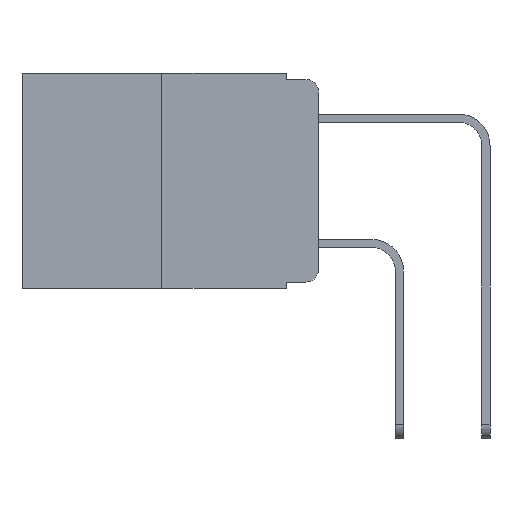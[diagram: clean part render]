
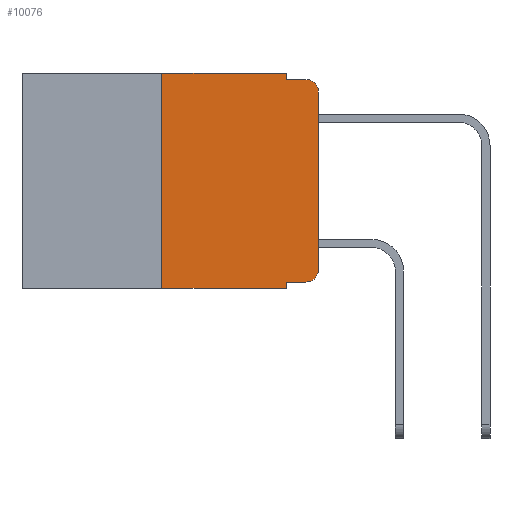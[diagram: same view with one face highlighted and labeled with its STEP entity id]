
A CAD part, left-side view. The second image highlights one B-rep face of the part: STEP entity #10076.
In plain terms, the highlighted planar face has unit normal (-1, 0, 0).
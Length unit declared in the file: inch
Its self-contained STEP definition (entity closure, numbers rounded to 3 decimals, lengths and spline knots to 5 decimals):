
#335 = DIRECTION ( 'NONE',  ( 0., -1., 0. ) ) ;
#600 = VERTEX_POINT ( 'NONE', #12245 ) ;
#879 = VERTEX_POINT ( 'NONE', #8091 ) ;
#1164 = VECTOR ( 'NONE', #9520, 39.37008 ) ;
#1260 = EDGE_CURVE ( 'NONE', #3278, #600, #9013, .T. ) ;
#1287 = CARTESIAN_POINT ( 'NONE',  ( 0., 0.051, 0. ) ) ;
#1298 = LINE ( 'NONE', #4380, #4053 ) ;
#1307 = VECTOR ( 'NONE', #12682, 39.37008 ) ;
#1690 = ORIENTED_EDGE ( 'NONE', *, *, #4685, .F. ) ;
#1772 = PLANE ( 'NONE',  #10299 ) ;
#1871 = CARTESIAN_POINT ( 'NONE',  ( 0., 0.02, -0.03 ) ) ;
#1982 = EDGE_CURVE ( 'NONE', #11834, #3278, #9294, .T. ) ;
#2088 = ORIENTED_EDGE ( 'NONE', *, *, #6685, .T. ) ;
#2178 = ORIENTED_EDGE ( 'NONE', *, *, #5344, .T. ) ;
#2198 = DIRECTION ( 'NONE',  ( -1., 0., 0. ) ) ;
#2210 = CARTESIAN_POINT ( 'NONE',  ( 0., 0.02, -0.313 ) ) ;
#2483 = CARTESIAN_POINT ( 'NONE',  ( 0., 0.25, 0. ) ) ;
#2591 = ORIENTED_EDGE ( 'NONE', *, *, #5039, .F. ) ;
#2690 = ORIENTED_EDGE ( 'NONE', *, *, #4041, .F. ) ;
#2692 = EDGE_CURVE ( 'NONE', #11834, #7189, #11748, .T. ) ;
#2758 = CARTESIAN_POINT ( 'NONE',  ( 0., 0.051, -0.333 ) ) ;
#2781 = ORIENTED_EDGE ( 'NONE', *, *, #1260, .T. ) ;
#2827 = EDGE_LOOP ( 'NONE', ( #2088, #2178, #1690, #2690, #2591, #6445, #5097, #8397, #3739, #2781 ) ) ;
#2858 = CARTESIAN_POINT ( 'NONE',  ( 0., 0.473, 0. ) ) ;
#2954 = DIRECTION ( 'NONE',  ( 0., 0., -1. ) ) ;
#3278 = VERTEX_POINT ( 'NONE', #11282 ) ;
#3390 = EDGE_CURVE ( 'NONE', #12925, #11996, #3933, .T. ) ;
#3414 = DIRECTION ( 'NONE',  ( 0., 0., -1. ) ) ;
#3492 = CARTESIAN_POINT ( 'NONE',  ( 0., 0.473, -0.343 ) ) ;
#3495 = VERTEX_POINT ( 'NONE', #11625 ) ;
#3739 = ORIENTED_EDGE ( 'NONE', *, *, #1982, .T. ) ;
#3858 = DIRECTION ( 'NONE',  ( 1., 0., 0. ) ) ;
#3933 = LINE ( 'NONE', #2483, #1164 ) ;
#3936 = CARTESIAN_POINT ( 'NONE',  ( 0., 0.051, 0. ) ) ;
#4041 = EDGE_CURVE ( 'NONE', #8054, #4931, #6684, .T. ) ;
#4053 = VECTOR ( 'NONE', #10375, 39.37008 ) ;
#4326 = CARTESIAN_POINT ( 'NONE',  ( 0., 0.051, -0.343 ) ) ;
#4380 = CARTESIAN_POINT ( 'NONE',  ( 0., 0.473, 0. ) ) ;
#4685 = EDGE_CURVE ( 'NONE', #4931, #879, #11849, .T. ) ;
#4931 = VERTEX_POINT ( 'NONE', #11191 ) ;
#5018 = CARTESIAN_POINT ( 'NONE',  ( 0., 0.25, 0. ) ) ;
#5039 = EDGE_CURVE ( 'NONE', #11996, #8054, #1298, .T. ) ;
#5097 = ORIENTED_EDGE ( 'NONE', *, *, #12477, .T. ) ;
#5344 = EDGE_CURVE ( 'NONE', #3495, #879, #10301, .T. ) ;
#5357 = CARTESIAN_POINT ( 'NONE',  ( 0., 0.25, -0.343 ) ) ;
#6403 = VECTOR ( 'NONE', #3414, 39.37008 ) ;
#6445 = ORIENTED_EDGE ( 'NONE', *, *, #3390, .F. ) ;
#6581 = VECTOR ( 'NONE', #10231, 39.37008 ) ;
#6684 = LINE ( 'NONE', #12639, #1307 ) ;
#6685 = EDGE_CURVE ( 'NONE', #600, #3495, #10144, .T. ) ;
#7189 = VERTEX_POINT ( 'NONE', #4326 ) ;
#7792 = CARTESIAN_POINT ( 'NONE',  ( 0., 0.051, -0.01 ) ) ;
#8054 = VERTEX_POINT ( 'NONE', #3936 ) ;
#8091 = CARTESIAN_POINT ( 'NONE',  ( 0., 0.02, -0.01 ) ) ;
#8179 = DIRECTION ( 'NONE',  ( 0., 0., -1. ) ) ;
#8397 = ORIENTED_EDGE ( 'NONE', *, *, #2692, .F. ) ;
#8826 = DIRECTION ( 'NONE',  ( 0., -1., 0. ) ) ;
#8921 = VECTOR ( 'NONE', #335, 39.37008 ) ;
#8952 = DIRECTION ( 'NONE',  ( -1., 0., 0. ) ) ;
#9013 = CIRCLE ( 'NONE', #11795, 0.02 ) ;
#9294 = LINE ( 'NONE', #10324, #6581 ) ;
#9520 = DIRECTION ( 'NONE',  ( 0., 0., 1. ) ) ;
#9543 = VECTOR ( 'NONE', #8826, 39.37008 ) ;
#10076 = ADVANCED_FACE ( 'NONE', ( #12962 ), #1772, .F. ) ;
#10144 = LINE ( 'NONE', #10728, #12450 ) ;
#10231 = DIRECTION ( 'NONE',  ( 0., -1., 0. ) ) ;
#10299 = AXIS2_PLACEMENT_3D ( 'NONE', #2858, #3858, #10834 ) ;
#10301 = CIRCLE ( 'NONE', #12900, 0.02 ) ;
#10324 = CARTESIAN_POINT ( 'NONE',  ( 0., 0.051, -0.333 ) ) ;
#10375 = DIRECTION ( 'NONE',  ( 0., -1., 0. ) ) ;
#10728 = CARTESIAN_POINT ( 'NONE',  ( 0., 0., 0. ) ) ;
#10834 = DIRECTION ( 'NONE',  ( 0., 0., -1. ) ) ;
#11191 = CARTESIAN_POINT ( 'NONE',  ( 0., 0.051, -0.01 ) ) ;
#11282 = CARTESIAN_POINT ( 'NONE',  ( 0., 0.02, -0.333 ) ) ;
#11540 = LINE ( 'NONE', #3492, #8921 ) ;
#11625 = CARTESIAN_POINT ( 'NONE',  ( 0., 0., -0.03 ) ) ;
#11722 = DIRECTION ( 'NONE',  ( 0., 0., 1. ) ) ;
#11748 = LINE ( 'NONE', #1287, #6403 ) ;
#11795 = AXIS2_PLACEMENT_3D ( 'NONE', #2210, #2198, #8179 ) ;
#11834 = VERTEX_POINT ( 'NONE', #2758 ) ;
#11849 = LINE ( 'NONE', #7792, #9543 ) ;
#11996 = VERTEX_POINT ( 'NONE', #5018 ) ;
#12245 = CARTESIAN_POINT ( 'NONE',  ( 0., 0., -0.313 ) ) ;
#12450 = VECTOR ( 'NONE', #11722, 39.37008 ) ;
#12477 = EDGE_CURVE ( 'NONE', #12925, #7189, #11540, .T. ) ;
#12639 = CARTESIAN_POINT ( 'NONE',  ( 0., 0.051, 0. ) ) ;
#12682 = DIRECTION ( 'NONE',  ( 0., 0., -1. ) ) ;
#12900 = AXIS2_PLACEMENT_3D ( 'NONE', #1871, #8952, #2954 ) ;
#12925 = VERTEX_POINT ( 'NONE', #5357 ) ;
#12962 = FACE_OUTER_BOUND ( 'NONE', #2827, .T. ) ;
